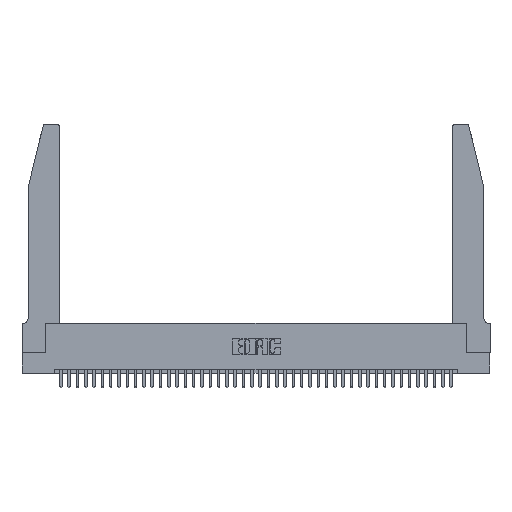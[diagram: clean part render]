
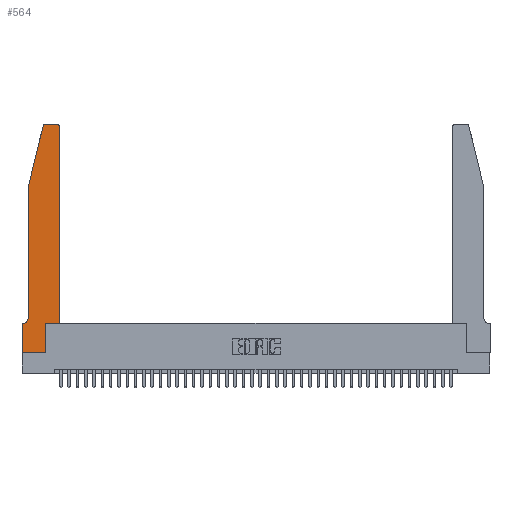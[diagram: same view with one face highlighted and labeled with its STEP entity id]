
A CAD part, top view. The second image highlights one B-rep face of the part: STEP entity #564.
In plain terms, the highlighted planar face has unit normal (0, 0, 1).
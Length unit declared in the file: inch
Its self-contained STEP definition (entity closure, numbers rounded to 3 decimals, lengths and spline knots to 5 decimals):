
#164 = DIRECTION ( 'NONE',  ( 0., 0., 1. ) ) ;
#413 = EDGE_CURVE ( 'NONE', #30145, #33849, #5347, .T. ) ;
#564 = ADVANCED_FACE ( 'NONE', ( #19916 ), #6802, .T. ) ;
#789 = CARTESIAN_POINT ( 'NONE',  ( 0.284, 2.72, 0.37 ) ) ;
#916 = DIRECTION ( 'NONE',  ( 1., 0., 0. ) ) ;
#968 = CARTESIAN_POINT ( 'NONE',  ( 0.4505, 0.35, 0.37 ) ) ;
#1476 = DIRECTION ( 'NONE',  ( 0., 0., 1. ) ) ;
#1591 = EDGE_CURVE ( 'NONE', #37839, #20696, #22335, .T. ) ;
#2454 = LINE ( 'NONE', #19915, #35696 ) ;
#2954 = ORIENTED_EDGE ( 'NONE', *, *, #40245, .T. ) ;
#2979 = CARTESIAN_POINT ( 'NONE',  ( 0.2865, 0., 0.37 ) ) ;
#3635 = CARTESIAN_POINT ( 'NONE',  ( 0.0755, 0.42, 0.37 ) ) ;
#3843 = CARTESIAN_POINT ( 'NONE',  ( 0.2605, 2.75, 0.37 ) ) ;
#4060 = VECTOR ( 'NONE', #23521, 39.37008 ) ;
#4673 = EDGE_CURVE ( 'NONE', #15791, #30145, #2454, .T. ) ;
#4737 = CARTESIAN_POINT ( 'NONE',  ( 0.4505, 2.72, 0.37 ) ) ;
#5262 = VECTOR ( 'NONE', #33227, 39.37008 ) ;
#5347 = LINE ( 'NONE', #6236, #32507 ) ;
#5592 = LINE ( 'NONE', #15234, #15158 ) ;
#6222 = EDGE_CURVE ( 'NONE', #39185, #37839, #21457, .T. ) ;
#6236 = CARTESIAN_POINT ( 'NONE',  ( 0.0755, 2., 0.37 ) ) ;
#6255 = AXIS2_PLACEMENT_3D ( 'NONE', #19327, #164, #32266 ) ;
#6525 = ORIENTED_EDGE ( 'NONE', *, *, #1591, .T. ) ;
#6802 = PLANE ( 'NONE',  #6255 ) ;
#6983 = ORIENTED_EDGE ( 'NONE', *, *, #4673, .T. ) ;
#7244 = EDGE_CURVE ( 'NONE', #22728, #15791, #15395, .T. ) ;
#7358 = VECTOR ( 'NONE', #27658, 39.37008 ) ;
#7819 = CARTESIAN_POINT ( 'NONE',  ( 0.0055, 0.35, 0.37 ) ) ;
#8792 = VECTOR ( 'NONE', #36125, 39.37008 ) ;
#8831 = ORIENTED_EDGE ( 'NONE', *, *, #28137, .T. ) ;
#9288 = VECTOR ( 'NONE', #14806, 39.37008 ) ;
#9784 = LINE ( 'NONE', #26835, #8792 ) ;
#10081 = ORIENTED_EDGE ( 'NONE', *, *, #32045, .T. ) ;
#11198 = DIRECTION ( 'NONE',  ( 1., 0., 0. ) ) ;
#11591 = VERTEX_POINT ( 'NONE', #7819 ) ;
#11877 = DIRECTION ( 'NONE',  ( 1., 0., 0. ) ) ;
#12312 = CARTESIAN_POINT ( 'NONE',  ( 0.0055, 0.42, 0.37 ) ) ;
#12642 = LINE ( 'NONE', #968, #4060 ) ;
#12727 = DIRECTION ( 'NONE',  ( 0., -1., 0. ) ) ;
#13693 = DIRECTION ( 'NONE',  ( -0.239, -0.971, 0. ) ) ;
#14570 = CARTESIAN_POINT ( 'NONE',  ( 0.284, 2.75, 0.37 ) ) ;
#14673 = CARTESIAN_POINT ( 'NONE',  ( 0., 0., 0.37 ) ) ;
#14691 = CARTESIAN_POINT ( 'NONE',  ( 0.2865, 0.35, 0.37 ) ) ;
#14806 = DIRECTION ( 'NONE',  ( 0., -1., 0. ) ) ;
#14940 = CARTESIAN_POINT ( 'NONE',  ( 0., 0., 0.37 ) ) ;
#15136 = ORIENTED_EDGE ( 'NONE', *, *, #6222, .T. ) ;
#15158 = VECTOR ( 'NONE', #11877, 39.37008 ) ;
#15234 = CARTESIAN_POINT ( 'NONE',  ( 0.4505, 0.35, 0.37 ) ) ;
#15395 = CIRCLE ( 'NONE', #22589, 0.03 ) ;
#15791 = VERTEX_POINT ( 'NONE', #30598 ) ;
#16665 = CARTESIAN_POINT ( 'NONE',  ( 0., 0., 0.37 ) ) ;
#17996 = CARTESIAN_POINT ( 'NONE',  ( 0., 0.35, 0.37 ) ) ;
#19327 = CARTESIAN_POINT ( 'NONE',  ( 0., 0.35, 0.37 ) ) ;
#19458 = ORIENTED_EDGE ( 'NONE', *, *, #413, .T. ) ;
#19915 = CARTESIAN_POINT ( 'NONE',  ( 0.0755, 2., 0.37 ) ) ;
#19916 = FACE_OUTER_BOUND ( 'NONE', #21520, .T. ) ;
#20050 = VERTEX_POINT ( 'NONE', #17996 ) ;
#20230 = DIRECTION ( 'NONE',  ( 0., 0., 1. ) ) ;
#20625 = EDGE_CURVE ( 'NONE', #11591, #20050, #9784, .T. ) ;
#20696 = VERTEX_POINT ( 'NONE', #14691 ) ;
#20946 = EDGE_CURVE ( 'NONE', #36174, #22728, #31414, .T. ) ;
#21220 = CARTESIAN_POINT ( 'NONE',  ( 0.2865, 0.35, 0.37 ) ) ;
#21457 = LINE ( 'NONE', #14673, #7358 ) ;
#21520 = EDGE_LOOP ( 'NONE', ( #33677, #28811, #6983, #19458, #10081, #22330, #8831, #15136, #6525, #31054, #2954, #22010 ) ) ;
#22010 = ORIENTED_EDGE ( 'NONE', *, *, #22692, .T. ) ;
#22330 = ORIENTED_EDGE ( 'NONE', *, *, #20625, .T. ) ;
#22335 = LINE ( 'NONE', #21220, #33926 ) ;
#22589 = AXIS2_PLACEMENT_3D ( 'NONE', #789, #20230, #916 ) ;
#22657 = AXIS2_PLACEMENT_3D ( 'NONE', #27274, #1476, #11198 ) ;
#22692 = EDGE_CURVE ( 'NONE', #27382, #36174, #23450, .T. ) ;
#22728 = VERTEX_POINT ( 'NONE', #14570 ) ;
#23450 = CIRCLE ( 'NONE', #22657, 0.03 ) ;
#23521 = DIRECTION ( 'NONE',  ( 0., 1., 0. ) ) ;
#25142 = DIRECTION ( 'NONE',  ( 0., 1., 0. ) ) ;
#25308 = AXIS2_PLACEMENT_3D ( 'NONE', #12312, #34961, #38214 ) ;
#25411 = CARTESIAN_POINT ( 'NONE',  ( 0.0755, 2., 0.37 ) ) ;
#26835 = CARTESIAN_POINT ( 'NONE',  ( 0.0755, 0.35, 0.37 ) ) ;
#27274 = CARTESIAN_POINT ( 'NONE',  ( 0.4205, 2.72, 0.37 ) ) ;
#27382 = VERTEX_POINT ( 'NONE', #4737 ) ;
#27658 = DIRECTION ( 'NONE',  ( 1., 0., 0. ) ) ;
#27687 = VERTEX_POINT ( 'NONE', #37808 ) ;
#28137 = EDGE_CURVE ( 'NONE', #20050, #39185, #41092, .T. ) ;
#28811 = ORIENTED_EDGE ( 'NONE', *, *, #7244, .T. ) ;
#30145 = VERTEX_POINT ( 'NONE', #25411 ) ;
#30598 = CARTESIAN_POINT ( 'NONE',  ( 0.25487, 2.72718, 0.37 ) ) ;
#31054 = ORIENTED_EDGE ( 'NONE', *, *, #34611, .T. ) ;
#31414 = LINE ( 'NONE', #3843, #5262 ) ;
#32045 = EDGE_CURVE ( 'NONE', #33849, #11591, #32167, .T. ) ;
#32167 = CIRCLE ( 'NONE', #25308, 0.07 ) ;
#32266 = DIRECTION ( 'NONE',  ( 1., 0., 0. ) ) ;
#32507 = VECTOR ( 'NONE', #12727, 39.37008 ) ;
#33227 = DIRECTION ( 'NONE',  ( -1., 0., 0. ) ) ;
#33677 = ORIENTED_EDGE ( 'NONE', *, *, #20946, .T. ) ;
#33849 = VERTEX_POINT ( 'NONE', #3635 ) ;
#33926 = VECTOR ( 'NONE', #25142, 39.37008 ) ;
#34611 = EDGE_CURVE ( 'NONE', #20696, #27687, #5592, .T. ) ;
#34961 = DIRECTION ( 'NONE',  ( 0., 0., -1. ) ) ;
#35696 = VECTOR ( 'NONE', #13693, 39.37008 ) ;
#36125 = DIRECTION ( 'NONE',  ( -1., 0., 0. ) ) ;
#36174 = VERTEX_POINT ( 'NONE', #36929 ) ;
#36929 = CARTESIAN_POINT ( 'NONE',  ( 0.4205, 2.75, 0.37 ) ) ;
#37808 = CARTESIAN_POINT ( 'NONE',  ( 0.4505, 0.35, 0.37 ) ) ;
#37839 = VERTEX_POINT ( 'NONE', #2979 ) ;
#38214 = DIRECTION ( 'NONE',  ( -1., 0., 0. ) ) ;
#39185 = VERTEX_POINT ( 'NONE', #16665 ) ;
#40245 = EDGE_CURVE ( 'NONE', #27687, #27382, #12642, .T. ) ;
#41092 = LINE ( 'NONE', #14940, #9288 ) ;
